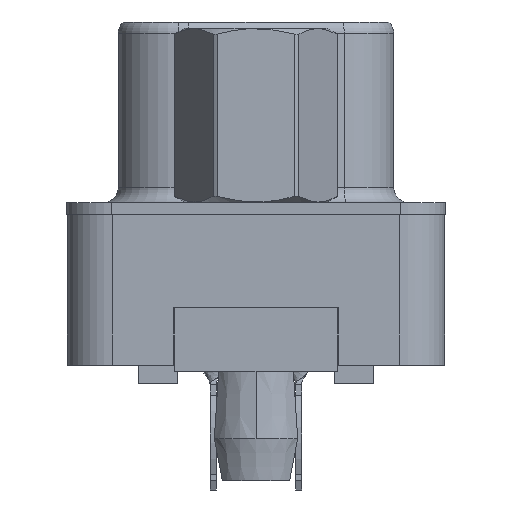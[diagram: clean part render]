
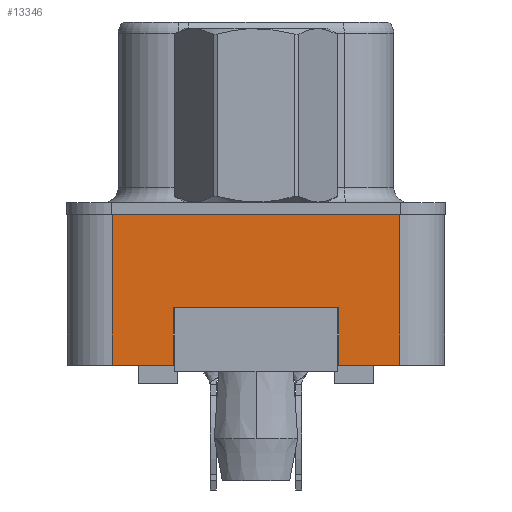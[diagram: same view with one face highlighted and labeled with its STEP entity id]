
A CAD part, left-side view. The second image highlights one B-rep face of the part: STEP entity #13346.
In plain terms, the highlighted planar face has unit normal (-1, 0, 0).
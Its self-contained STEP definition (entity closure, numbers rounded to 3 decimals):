
#613 = VECTOR ( 'NONE', #2017, 1000. ) ;
#1435 = LINE ( 'NONE', #8112, #15411 ) ;
#1729 = LINE ( 'NONE', #19127, #613 ) ;
#2017 = DIRECTION ( 'NONE',  ( 0., 0., -1. ) ) ;
#2062 = CARTESIAN_POINT ( 'NONE',  ( -3., 4.775, -5. ) ) ;
#2451 = CARTESIAN_POINT ( 'NONE',  ( -3., 4.775, 0. ) ) ;
#2549 = AXIS2_PLACEMENT_3D ( 'NONE', #18595, #27639, #16798 ) ;
#2626 = CARTESIAN_POINT ( 'NONE',  ( -3., -4.775, 0. ) ) ;
#3065 = DIRECTION ( 'NONE',  ( 0., -1., 0. ) ) ;
#3415 = VERTEX_POINT ( 'NONE', #22676 ) ;
#3834 = VECTOR ( 'NONE', #20264, 1000. ) ;
#4832 = VERTEX_POINT ( 'NONE', #2626 ) ;
#4928 = DIRECTION ( 'NONE',  ( 0., 1., 0. ) ) ;
#5070 = PLANE ( 'NONE',  #2549 ) ;
#5376 = VECTOR ( 'NONE', #4928, 1000. ) ;
#5484 = ORIENTED_EDGE ( 'NONE', *, *, #18859, .T. ) ;
#6162 = ORIENTED_EDGE ( 'NONE', *, *, #18619, .F. ) ;
#6522 = VERTEX_POINT ( 'NONE', #2451 ) ;
#7579 = FACE_OUTER_BOUND ( 'NONE', #8604, .T. ) ;
#7613 = ORIENTED_EDGE ( 'NONE', *, *, #15327, .T. ) ;
#7754 = VECTOR ( 'NONE', #3065, 1000. ) ;
#8112 = CARTESIAN_POINT ( 'NONE',  ( -3., -4.775, -5. ) ) ;
#8604 = EDGE_LOOP ( 'NONE', ( #10601, #7613, #11142, #6162, #10809, #5484, #17793, #26425 ) ) ;
#9088 = VECTOR ( 'NONE', #13753, 1000. ) ;
#9849 = VERTEX_POINT ( 'NONE', #16850 ) ;
#9974 = CARTESIAN_POINT ( 'NONE',  ( -3., -4.775, -5. ) ) ;
#10124 = LINE ( 'NONE', #9974, #9088 ) ;
#10601 = ORIENTED_EDGE ( 'NONE', *, *, #27776, .T. ) ;
#10675 = VERTEX_POINT ( 'NONE', #28351 ) ;
#10809 = ORIENTED_EDGE ( 'NONE', *, *, #23707, .F. ) ;
#11142 = ORIENTED_EDGE ( 'NONE', *, *, #24211, .T. ) ;
#11905 = CARTESIAN_POINT ( 'NONE',  ( -3., 2.75, -5. ) ) ;
#12419 = CARTESIAN_POINT ( 'NONE',  ( -3., -4.775, 0. ) ) ;
#13315 = CARTESIAN_POINT ( 'NONE',  ( -3., -2.75, -5. ) ) ;
#13346 = ADVANCED_FACE ( 'NONE', ( #7579 ), #5070, .T. ) ;
#13753 = DIRECTION ( 'NONE',  ( 0., 0., 1. ) ) ;
#14753 = VECTOR ( 'NONE', #27162, 1000. ) ;
#15106 = DIRECTION ( 'NONE',  ( 0., -1., 0. ) ) ;
#15301 = LINE ( 'NONE', #2062, #14753 ) ;
#15327 = EDGE_CURVE ( 'NONE', #18831, #3415, #1435, .T. ) ;
#15411 = VECTOR ( 'NONE', #24027, 1000. ) ;
#16798 = DIRECTION ( 'NONE',  ( 0., 0., 1. ) ) ;
#16850 = CARTESIAN_POINT ( 'NONE',  ( -3., 4.775, -5. ) ) ;
#17793 = ORIENTED_EDGE ( 'NONE', *, *, #25136, .F. ) ;
#18318 = CARTESIAN_POINT ( 'NONE',  ( -3., 2.75, -3.1 ) ) ;
#18595 = CARTESIAN_POINT ( 'NONE',  ( -3., -4.775, -5. ) ) ;
#18619 = EDGE_CURVE ( 'NONE', #6522, #4832, #21170, .T. ) ;
#18831 = VERTEX_POINT ( 'NONE', #13315 ) ;
#18859 = EDGE_CURVE ( 'NONE', #9849, #27206, #20137, .T. ) ;
#19127 = CARTESIAN_POINT ( 'NONE',  ( -3., -2.75, -3.1 ) ) ;
#20137 = LINE ( 'NONE', #28901, #27238 ) ;
#20264 = DIRECTION ( 'NONE',  ( 0., 0., -1. ) ) ;
#21170 = LINE ( 'NONE', #12419, #7754 ) ;
#22676 = CARTESIAN_POINT ( 'NONE',  ( -3., -4.775, -5. ) ) ;
#23610 = VERTEX_POINT ( 'NONE', #28655 ) ;
#23707 = EDGE_CURVE ( 'NONE', #9849, #6522, #15301, .T. ) ;
#24027 = DIRECTION ( 'NONE',  ( 0., -1., 0. ) ) ;
#24211 = EDGE_CURVE ( 'NONE', #3415, #4832, #10124, .T. ) ;
#24718 = LINE ( 'NONE', #25156, #3834 ) ;
#24839 = LINE ( 'NONE', #18318, #5376 ) ;
#25136 = EDGE_CURVE ( 'NONE', #10675, #27206, #24718, .T. ) ;
#25156 = CARTESIAN_POINT ( 'NONE',  ( -3., 2.75, -3.1 ) ) ;
#26425 = ORIENTED_EDGE ( 'NONE', *, *, #28323, .F. ) ;
#27162 = DIRECTION ( 'NONE',  ( 0., 0., 1. ) ) ;
#27206 = VERTEX_POINT ( 'NONE', #11905 ) ;
#27238 = VECTOR ( 'NONE', #15106, 1000. ) ;
#27639 = DIRECTION ( 'NONE',  ( -1., 0., 0. ) ) ;
#27776 = EDGE_CURVE ( 'NONE', #23610, #18831, #1729, .T. ) ;
#28323 = EDGE_CURVE ( 'NONE', #23610, #10675, #24839, .T. ) ;
#28351 = CARTESIAN_POINT ( 'NONE',  ( -3., 2.75, -3.1 ) ) ;
#28655 = CARTESIAN_POINT ( 'NONE',  ( -3., -2.75, -3.1 ) ) ;
#28901 = CARTESIAN_POINT ( 'NONE',  ( -3., -4.775, -5. ) ) ;
